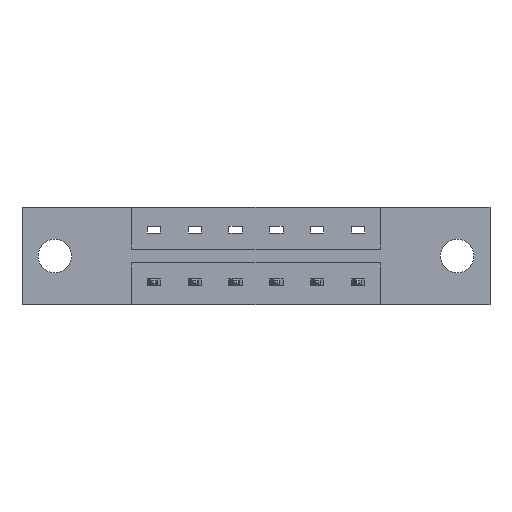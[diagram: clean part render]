
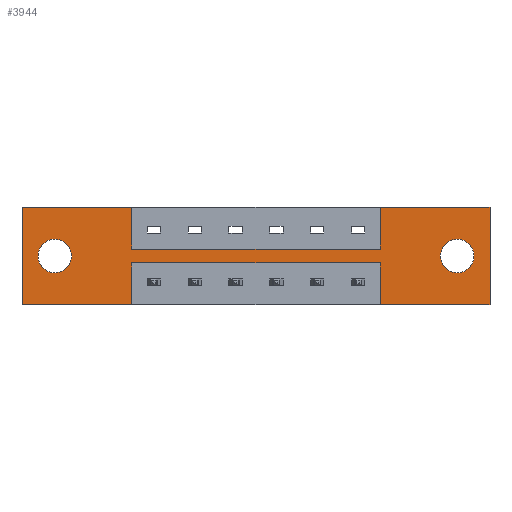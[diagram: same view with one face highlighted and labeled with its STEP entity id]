
A CAD part, front view. The second image highlights one B-rep face of the part: STEP entity #3944.
In plain terms, the highlighted planar face has unit normal (0, -1, 0).
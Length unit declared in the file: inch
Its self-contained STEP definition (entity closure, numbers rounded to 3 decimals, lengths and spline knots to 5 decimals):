
#78 = VERTEX_POINT ( 'NONE', #767 ) ;
#115 = VERTEX_POINT ( 'NONE', #1837 ) ;
#141 = DIRECTION ( 'NONE',  ( -1., 0., 0. ) ) ;
#194 = CARTESIAN_POINT ( 'NONE',  ( 1.659, 0., -0.185 ) ) ;
#242 = VERTEX_POINT ( 'NONE', #2887 ) ;
#250 = EDGE_CURVE ( 'NONE', #1815, #2432, #4166, .T. ) ;
#270 = CARTESIAN_POINT ( 'NONE',  ( 0., 0., 0. ) ) ;
#288 = CARTESIAN_POINT ( 'NONE',  ( 0., 0., 0. ) ) ;
#291 = VECTOR ( 'NONE', #6757, 39.37008 ) ;
#342 = DIRECTION ( 'NONE',  ( 0., 0., 1. ) ) ;
#423 = CIRCLE ( 'NONE', #2716, 0.064 ) ;
#508 = EDGE_CURVE ( 'NONE', #78, #3718, #3862, .T. ) ;
#716 = DIRECTION ( 'NONE',  ( 0., 0., -1. ) ) ;
#767 = CARTESIAN_POINT ( 'NONE',  ( 1.3665, 0., -0.1585 ) ) ;
#854 = FACE_BOUND ( 'NONE', #6223, .T. ) ;
#932 = CARTESIAN_POINT ( 'NONE',  ( 1.784, 0., 0. ) ) ;
#1105 = VECTOR ( 'NONE', #4490, 39.37008 ) ;
#1121 = EDGE_LOOP ( 'NONE', ( #6267, #2775 ) ) ;
#1125 = ORIENTED_EDGE ( 'NONE', *, *, #5549, .F. ) ;
#1150 = ORIENTED_EDGE ( 'NONE', *, *, #8004, .F. ) ;
#1221 = CIRCLE ( 'NONE', #5947, 0.064 ) ;
#1222 = LINE ( 'NONE', #5748, #1105 ) ;
#1296 = DIRECTION ( 'NONE',  ( -1., 0., 0. ) ) ;
#1449 = CARTESIAN_POINT ( 'NONE',  ( 1.3665, 0., -0.2115 ) ) ;
#1501 = CARTESIAN_POINT ( 'NONE',  ( 0.4175, 0., -0.1585 ) ) ;
#1506 = VERTEX_POINT ( 'NONE', #270 ) ;
#1519 = ORIENTED_EDGE ( 'NONE', *, *, #3057, .F. ) ;
#1608 = FACE_BOUND ( 'NONE', #1121, .T. ) ;
#1716 = DIRECTION ( 'NONE',  ( 0., 1., 0. ) ) ;
#1815 = VERTEX_POINT ( 'NONE', #932 ) ;
#1837 = CARTESIAN_POINT ( 'NONE',  ( 0.125, 0., -0.249 ) ) ;
#1910 = EDGE_CURVE ( 'NONE', #7903, #78, #5444, .T. ) ;
#2032 = LINE ( 'NONE', #7145, #7269 ) ;
#2051 = VERTEX_POINT ( 'NONE', #2990 ) ;
#2112 = CARTESIAN_POINT ( 'NONE',  ( 0., 0., -0.37 ) ) ;
#2411 = DIRECTION ( 'NONE',  ( -1., 0., 0. ) ) ;
#2432 = VERTEX_POINT ( 'NONE', #5712 ) ;
#2530 = VERTEX_POINT ( 'NONE', #7687 ) ;
#2572 = CARTESIAN_POINT ( 'NONE',  ( 0., 0., -0.37 ) ) ;
#2593 = ORIENTED_EDGE ( 'NONE', *, *, #6925, .T. ) ;
#2631 = VECTOR ( 'NONE', #4251, 39.37008 ) ;
#2657 = CARTESIAN_POINT ( 'NONE',  ( 1.3665, 0., -0.1585 ) ) ;
#2682 = CARTESIAN_POINT ( 'NONE',  ( 0., 0., -0.37 ) ) ;
#2695 = ORIENTED_EDGE ( 'NONE', *, *, #7830, .F. ) ;
#2696 = DIRECTION ( 'NONE',  ( 0., 0., 1. ) ) ;
#2716 = AXIS2_PLACEMENT_3D ( 'NONE', #194, #3340, #3468 ) ;
#2775 = ORIENTED_EDGE ( 'NONE', *, *, #7115, .T. ) ;
#2878 = ORIENTED_EDGE ( 'NONE', *, *, #508, .F. ) ;
#2887 = CARTESIAN_POINT ( 'NONE',  ( 0.125, 0., -0.121 ) ) ;
#2912 = DIRECTION ( 'NONE',  ( 0., 1., 0. ) ) ;
#2957 = LINE ( 'NONE', #288, #291 ) ;
#2975 = CIRCLE ( 'NONE', #6606, 0.064 ) ;
#2981 = CARTESIAN_POINT ( 'NONE',  ( 1.3665, 0., 0. ) ) ;
#2990 = CARTESIAN_POINT ( 'NONE',  ( 0.4175, 0., -0.2115 ) ) ;
#3001 = DIRECTION ( 'NONE',  ( 0., 0., -1. ) ) ;
#3057 = EDGE_CURVE ( 'NONE', #2432, #2530, #6618, .T. ) ;
#3102 = CARTESIAN_POINT ( 'NONE',  ( 0., 0., 0. ) ) ;
#3148 = LINE ( 'NONE', #6389, #5129 ) ;
#3340 = DIRECTION ( 'NONE',  ( 0., 1., 0. ) ) ;
#3399 = PLANE ( 'NONE',  #6073 ) ;
#3407 = VERTEX_POINT ( 'NONE', #1449 ) ;
#3468 = DIRECTION ( 'NONE',  ( 0., 0., -1. ) ) ;
#3483 = FACE_OUTER_BOUND ( 'NONE', #6006, .T. ) ;
#3574 = CARTESIAN_POINT ( 'NONE',  ( 1.659, 0., -0.121 ) ) ;
#3674 = CARTESIAN_POINT ( 'NONE',  ( 1.659, 0., -0.249 ) ) ;
#3718 = VERTEX_POINT ( 'NONE', #2981 ) ;
#3806 = AXIS2_PLACEMENT_3D ( 'NONE', #4234, #2912, #3001 ) ;
#3862 = LINE ( 'NONE', #2657, #4541 ) ;
#3938 = VECTOR ( 'NONE', #141, 39.37008 ) ;
#3944 = ADVANCED_FACE ( 'NONE', ( #854, #1608, #3483 ), #3399, .T. ) ;
#4099 = CARTESIAN_POINT ( 'NONE',  ( 0.4175, 0., -0.37 ) ) ;
#4166 = LINE ( 'NONE', #8068, #2631 ) ;
#4234 = CARTESIAN_POINT ( 'NONE',  ( 1.659, 0., -0.185 ) ) ;
#4251 = DIRECTION ( 'NONE',  ( 0., 0., -1. ) ) ;
#4311 = DIRECTION ( 'NONE',  ( 0., 0., 1. ) ) ;
#4360 = VERTEX_POINT ( 'NONE', #3674 ) ;
#4490 = DIRECTION ( 'NONE',  ( 1., 0., 0. ) ) ;
#4518 = LINE ( 'NONE', #7205, #3938 ) ;
#4541 = VECTOR ( 'NONE', #2696, 39.37008 ) ;
#4580 = VECTOR ( 'NONE', #716, 39.37008 ) ;
#4746 = ORIENTED_EDGE ( 'NONE', *, *, #5083, .F. ) ;
#4760 = CARTESIAN_POINT ( 'NONE',  ( 0.4175, 0., -0.2115 ) ) ;
#5051 = DIRECTION ( 'NONE',  ( 1., 0., 0. ) ) ;
#5083 = EDGE_CURVE ( 'NONE', #2530, #3407, #2032, .T. ) ;
#5129 = VECTOR ( 'NONE', #2411, 39.37008 ) ;
#5149 = CARTESIAN_POINT ( 'NONE',  ( 0.125, 0., -0.185 ) ) ;
#5231 = VECTOR ( 'NONE', #6065, 39.37008 ) ;
#5261 = VECTOR ( 'NONE', #5051, 39.37008 ) ;
#5292 = LINE ( 'NONE', #5754, #4580 ) ;
#5378 = DIRECTION ( 'NONE',  ( 0., 0., -1. ) ) ;
#5444 = LINE ( 'NONE', #1501, #5231 ) ;
#5461 = EDGE_CURVE ( 'NONE', #3718, #1815, #8200, .T. ) ;
#5471 = EDGE_CURVE ( 'NONE', #7437, #6623, #3148, .T. ) ;
#5518 = ORIENTED_EDGE ( 'NONE', *, *, #250, .F. ) ;
#5549 = EDGE_CURVE ( 'NONE', #7180, #7903, #5292, .T. ) ;
#5552 = CIRCLE ( 'NONE', #3806, 0.064 ) ;
#5575 = ORIENTED_EDGE ( 'NONE', *, *, #5461, .F. ) ;
#5599 = CARTESIAN_POINT ( 'NONE',  ( 0.125, 0., -0.185 ) ) ;
#5712 = CARTESIAN_POINT ( 'NONE',  ( 1.784, 0., -0.37 ) ) ;
#5748 = CARTESIAN_POINT ( 'NONE',  ( 0., 0., 0. ) ) ;
#5754 = CARTESIAN_POINT ( 'NONE',  ( 0.4175, 0., -0.1585 ) ) ;
#5801 = DIRECTION ( 'NONE',  ( 0., 0., 1. ) ) ;
#5947 = AXIS2_PLACEMENT_3D ( 'NONE', #5149, #1716, #4311 ) ;
#6006 = EDGE_LOOP ( 'NONE', ( #4746, #1519, #5518, #5575, #2878, #7661, #1125, #1150, #7642, #6302, #2695, #6084 ) ) ;
#6065 = DIRECTION ( 'NONE',  ( 1., 0., 0. ) ) ;
#6073 = AXIS2_PLACEMENT_3D ( 'NONE', #2112, #7273, #5378 ) ;
#6084 = ORIENTED_EDGE ( 'NONE', *, *, #7217, .F. ) ;
#6092 = EDGE_CURVE ( 'NONE', #242, #115, #2975, .T. ) ;
#6223 = EDGE_LOOP ( 'NONE', ( #2593, #8341 ) ) ;
#6267 = ORIENTED_EDGE ( 'NONE', *, *, #6092, .T. ) ;
#6302 = ORIENTED_EDGE ( 'NONE', *, *, #5471, .F. ) ;
#6367 = VECTOR ( 'NONE', #1296, 39.37008 ) ;
#6389 = CARTESIAN_POINT ( 'NONE',  ( 0., 0., -0.37 ) ) ;
#6606 = AXIS2_PLACEMENT_3D ( 'NONE', #5599, #6855, #342 ) ;
#6618 = LINE ( 'NONE', #2682, #6367 ) ;
#6623 = VERTEX_POINT ( 'NONE', #2572 ) ;
#6757 = DIRECTION ( 'NONE',  ( 0., 0., 1. ) ) ;
#6855 = DIRECTION ( 'NONE',  ( 0., 1., 0. ) ) ;
#6925 = EDGE_CURVE ( 'NONE', #7740, #4360, #5552, .T. ) ;
#7115 = EDGE_CURVE ( 'NONE', #115, #242, #1221, .T. ) ;
#7117 = CARTESIAN_POINT ( 'NONE',  ( 0.4175, 0., 0. ) ) ;
#7145 = CARTESIAN_POINT ( 'NONE',  ( 1.3665, 0., -0.2115 ) ) ;
#7180 = VERTEX_POINT ( 'NONE', #7117 ) ;
#7205 = CARTESIAN_POINT ( 'NONE',  ( 0.4175, 0., -0.2115 ) ) ;
#7217 = EDGE_CURVE ( 'NONE', #3407, #2051, #4518, .T. ) ;
#7269 = VECTOR ( 'NONE', #5801, 39.37008 ) ;
#7273 = DIRECTION ( 'NONE',  ( 0., -1., 0. ) ) ;
#7281 = LINE ( 'NONE', #4760, #7453 ) ;
#7437 = VERTEX_POINT ( 'NONE', #4099 ) ;
#7453 = VECTOR ( 'NONE', #7905, 39.37008 ) ;
#7642 = ORIENTED_EDGE ( 'NONE', *, *, #8208, .F. ) ;
#7661 = ORIENTED_EDGE ( 'NONE', *, *, #1910, .F. ) ;
#7687 = CARTESIAN_POINT ( 'NONE',  ( 1.3665, 0., -0.37 ) ) ;
#7740 = VERTEX_POINT ( 'NONE', #3574 ) ;
#7761 = CARTESIAN_POINT ( 'NONE',  ( 0.4175, 0., -0.1585 ) ) ;
#7830 = EDGE_CURVE ( 'NONE', #2051, #7437, #7281, .T. ) ;
#7903 = VERTEX_POINT ( 'NONE', #7761 ) ;
#7905 = DIRECTION ( 'NONE',  ( 0., 0., -1. ) ) ;
#8004 = EDGE_CURVE ( 'NONE', #1506, #7180, #1222, .T. ) ;
#8068 = CARTESIAN_POINT ( 'NONE',  ( 1.784, 0., 0. ) ) ;
#8145 = EDGE_CURVE ( 'NONE', #4360, #7740, #423, .T. ) ;
#8200 = LINE ( 'NONE', #3102, #5261 ) ;
#8208 = EDGE_CURVE ( 'NONE', #6623, #1506, #2957, .T. ) ;
#8341 = ORIENTED_EDGE ( 'NONE', *, *, #8145, .T. ) ;
